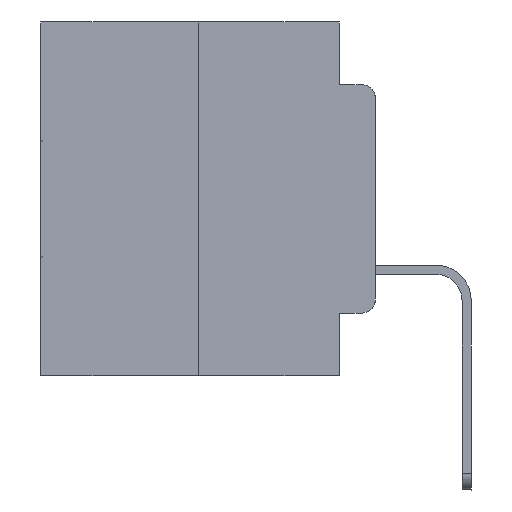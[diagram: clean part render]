
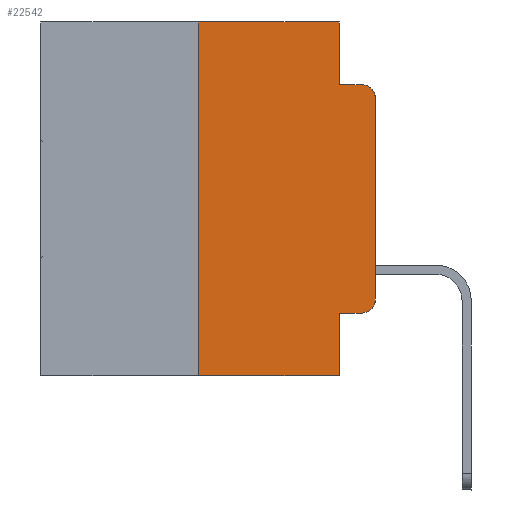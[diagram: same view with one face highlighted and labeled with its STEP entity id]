
A CAD part, left-side view. The second image highlights one B-rep face of the part: STEP entity #22542.
In plain terms, the highlighted planar face has unit normal (-1, 0, 0).
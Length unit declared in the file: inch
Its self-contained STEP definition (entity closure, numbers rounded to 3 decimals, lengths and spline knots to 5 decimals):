
#34 = CARTESIAN_POINT ( 'NONE',  ( 0., 0.051, 0. ) ) ;
#261 = DIRECTION ( 'NONE',  ( 0., -1., 0. ) ) ;
#511 = EDGE_CURVE ( 'NONE', #23771, #2370, #22416, .T. ) ;
#725 = LINE ( 'NONE', #23366, #10570 ) ;
#985 = EDGE_CURVE ( 'NONE', #13492, #29169, #4420, .T. ) ;
#1567 = CARTESIAN_POINT ( 'NONE',  ( 0., 0.02, -0.3915 ) ) ;
#2018 = CARTESIAN_POINT ( 'NONE',  ( 0., 0.473, -0.5 ) ) ;
#2330 = CARTESIAN_POINT ( 'NONE',  ( 0., 0.051, -0.4115 ) ) ;
#2370 = VERTEX_POINT ( 'NONE', #11822 ) ;
#2751 = VECTOR ( 'NONE', #6336, 39.37008 ) ;
#3073 = EDGE_CURVE ( 'NONE', #5103, #20599, #9253, .T. ) ;
#3208 = AXIS2_PLACEMENT_3D ( 'NONE', #1567, #23907, #12988 ) ;
#3575 = ORIENTED_EDGE ( 'NONE', *, *, #7134, .F. ) ;
#3783 = DIRECTION ( 'NONE',  ( 0., 0., -1. ) ) ;
#3886 = EDGE_CURVE ( 'NONE', #9609, #23771, #725, .T. ) ;
#4103 = DIRECTION ( 'NONE',  ( 0., -1., 0. ) ) ;
#4356 = CARTESIAN_POINT ( 'NONE',  ( 0., 0.051, -0.5 ) ) ;
#4420 = LINE ( 'NONE', #19072, #12122 ) ;
#4511 = CARTESIAN_POINT ( 'NONE',  ( 0., 0.051, -0.0885 ) ) ;
#5103 = VERTEX_POINT ( 'NONE', #24358 ) ;
#5762 = CIRCLE ( 'NONE', #3208, 0.02 ) ;
#6336 = DIRECTION ( 'NONE',  ( 0., 0., -1. ) ) ;
#6870 = EDGE_CURVE ( 'NONE', #9460, #23450, #10073, .T. ) ;
#7048 = DIRECTION ( 'NONE',  ( 0., 0., 1. ) ) ;
#7134 = EDGE_CURVE ( 'NONE', #2370, #18651, #27338, .T. ) ;
#7170 = DIRECTION ( 'NONE',  ( 1., 0., 0. ) ) ;
#7229 = CARTESIAN_POINT ( 'NONE',  ( 0., 0.25, 0. ) ) ;
#7815 = CARTESIAN_POINT ( 'NONE',  ( 0., 0., -0.1085 ) ) ;
#7995 = VECTOR ( 'NONE', #7048, 39.37008 ) ;
#8798 = ORIENTED_EDGE ( 'NONE', *, *, #985, .T. ) ;
#9253 = LINE ( 'NONE', #2330, #20522 ) ;
#9392 = VECTOR ( 'NONE', #4103, 39.37008 ) ;
#9460 = VERTEX_POINT ( 'NONE', #21901 ) ;
#9609 = VERTEX_POINT ( 'NONE', #7229 ) ;
#9649 = CIRCLE ( 'NONE', #27522, 0.02 ) ;
#10073 = LINE ( 'NONE', #2018, #9392 ) ;
#10369 = EDGE_CURVE ( 'NONE', #29169, #18651, #9649, .T. ) ;
#10570 = VECTOR ( 'NONE', #20811, 39.37008 ) ;
#11822 = CARTESIAN_POINT ( 'NONE',  ( 0., 0.051, -0.0885 ) ) ;
#12122 = VECTOR ( 'NONE', #12346, 39.37008 ) ;
#12346 = DIRECTION ( 'NONE',  ( 0., 0., 1. ) ) ;
#12490 = CARTESIAN_POINT ( 'NONE',  ( 0., 0.051, 0. ) ) ;
#12988 = DIRECTION ( 'NONE',  ( 0., 0., -1. ) ) ;
#13492 = VERTEX_POINT ( 'NONE', #23519 ) ;
#13695 = ORIENTED_EDGE ( 'NONE', *, *, #24469, .F. ) ;
#14424 = EDGE_CURVE ( 'NONE', #9460, #9609, #20706, .T. ) ;
#14995 = VECTOR ( 'NONE', #3783, 39.37008 ) ;
#18054 = ORIENTED_EDGE ( 'NONE', *, *, #10369, .T. ) ;
#18337 = ORIENTED_EDGE ( 'NONE', *, *, #14424, .F. ) ;
#18412 = CARTESIAN_POINT ( 'NONE',  ( 0., 0.473, 0. ) ) ;
#18651 = VERTEX_POINT ( 'NONE', #22219 ) ;
#19072 = CARTESIAN_POINT ( 'NONE',  ( 0., 0., 0. ) ) ;
#19190 = ORIENTED_EDGE ( 'NONE', *, *, #3886, .F. ) ;
#19449 = CARTESIAN_POINT ( 'NONE',  ( 0., 0.051, 0. ) ) ;
#19858 = EDGE_CURVE ( 'NONE', #20599, #13492, #5762, .T. ) ;
#19971 = DIRECTION ( 'NONE',  ( 0., 0., -1. ) ) ;
#20522 = VECTOR ( 'NONE', #29184, 39.37008 ) ;
#20599 = VERTEX_POINT ( 'NONE', #26730 ) ;
#20706 = LINE ( 'NONE', #27122, #7995 ) ;
#20811 = DIRECTION ( 'NONE',  ( 0., -1., 0. ) ) ;
#21696 = ORIENTED_EDGE ( 'NONE', *, *, #6870, .T. ) ;
#21901 = CARTESIAN_POINT ( 'NONE',  ( 0., 0.25, -0.5 ) ) ;
#21924 = AXIS2_PLACEMENT_3D ( 'NONE', #18412, #7170, #25172 ) ;
#22219 = CARTESIAN_POINT ( 'NONE',  ( 0., 0.02, -0.0885 ) ) ;
#22416 = LINE ( 'NONE', #19449, #14995 ) ;
#22542 = ADVANCED_FACE ( 'NONE', ( #23249 ), #27530, .F. ) ;
#22841 = LINE ( 'NONE', #34, #2751 ) ;
#23116 = ORIENTED_EDGE ( 'NONE', *, *, #511, .F. ) ;
#23249 = FACE_OUTER_BOUND ( 'NONE', #26785, .T. ) ;
#23366 = CARTESIAN_POINT ( 'NONE',  ( 0., 0.473, 0. ) ) ;
#23450 = VERTEX_POINT ( 'NONE', #4356 ) ;
#23519 = CARTESIAN_POINT ( 'NONE',  ( 0., 0., -0.3915 ) ) ;
#23771 = VERTEX_POINT ( 'NONE', #12490 ) ;
#23907 = DIRECTION ( 'NONE',  ( -1., 0., 0. ) ) ;
#24358 = CARTESIAN_POINT ( 'NONE',  ( 0., 0.051, -0.4115 ) ) ;
#24469 = EDGE_CURVE ( 'NONE', #5103, #23450, #22841, .T. ) ;
#25172 = DIRECTION ( 'NONE',  ( 0., 0., -1. ) ) ;
#25541 = ORIENTED_EDGE ( 'NONE', *, *, #19858, .T. ) ;
#25732 = ORIENTED_EDGE ( 'NONE', *, *, #3073, .T. ) ;
#26645 = CARTESIAN_POINT ( 'NONE',  ( 0., 0.02, -0.1085 ) ) ;
#26730 = CARTESIAN_POINT ( 'NONE',  ( 0., 0.02, -0.4115 ) ) ;
#26785 = EDGE_LOOP ( 'NONE', ( #8798, #18054, #3575, #23116, #19190, #18337, #21696, #13695, #25732, #25541 ) ) ;
#27122 = CARTESIAN_POINT ( 'NONE',  ( 0., 0.25, 0. ) ) ;
#27338 = LINE ( 'NONE', #4511, #28035 ) ;
#27522 = AXIS2_PLACEMENT_3D ( 'NONE', #26645, #28922, #19971 ) ;
#27530 = PLANE ( 'NONE',  #21924 ) ;
#28035 = VECTOR ( 'NONE', #261, 39.37008 ) ;
#28922 = DIRECTION ( 'NONE',  ( -1., 0., 0. ) ) ;
#29169 = VERTEX_POINT ( 'NONE', #7815 ) ;
#29184 = DIRECTION ( 'NONE',  ( 0., -1., 0. ) ) ;
